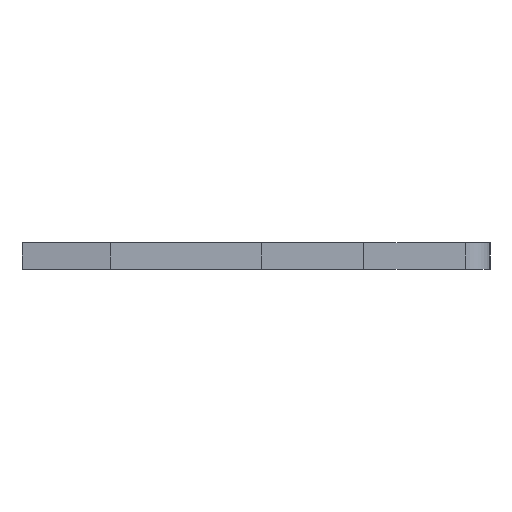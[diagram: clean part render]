
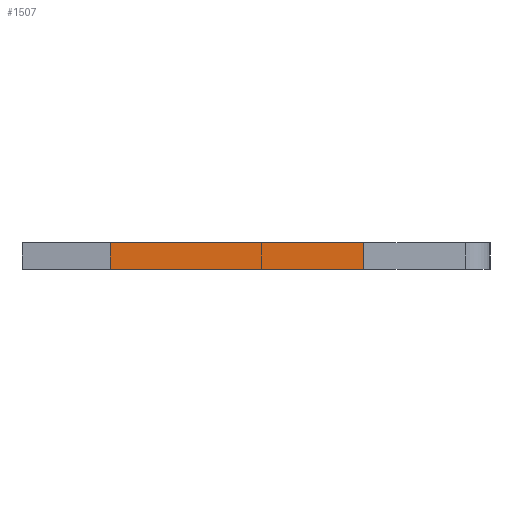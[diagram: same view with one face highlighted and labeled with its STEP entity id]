
A CAD part, left-side view. The second image highlights one B-rep face of the part: STEP entity #1507.
In plain terms, the highlighted face is planar.
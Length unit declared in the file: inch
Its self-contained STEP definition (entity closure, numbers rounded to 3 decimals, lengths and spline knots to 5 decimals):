
#182 = ORIENTED_EDGE ( 'NONE', *, *, #1383, .F. ) ;
#221 = CARTESIAN_POINT ( 'NONE',  ( 0.013, -0.099, -0.0575 ) ) ;
#313 = EDGE_LOOP ( 'NONE', ( #1690, #182, #1790, #849 ) ) ;
#319 = DIRECTION ( 'NONE',  ( 0., 1., 0. ) ) ;
#337 = CARTESIAN_POINT ( 'NONE',  ( -0.013, 0.146, -0.0575 ) ) ;
#366 = CARTESIAN_POINT ( 'NONE',  ( 0.013, 0.146, -0.0575 ) ) ;
#397 = DIRECTION ( 'NONE',  ( -1., 0., 0. ) ) ;
#422 = FACE_OUTER_BOUND ( 'NONE', #313, .T. ) ;
#446 = VECTOR ( 'NONE', #1350, 39.37008 ) ;
#530 = VERTEX_POINT ( 'NONE', #821 ) ;
#560 = DIRECTION ( 'NONE',  ( 1., 0., 0. ) ) ;
#689 = CARTESIAN_POINT ( 'NONE',  ( 0.013, -0.099, -0.0575 ) ) ;
#758 = VERTEX_POINT ( 'NONE', #1055 ) ;
#782 = VECTOR ( 'NONE', #1108, 39.37008 ) ;
#784 = EDGE_CURVE ( 'NONE', #2197, #758, #1020, .T. ) ;
#821 = CARTESIAN_POINT ( 'NONE',  ( 0.013, 0.146, -0.0575 ) ) ;
#849 = ORIENTED_EDGE ( 'NONE', *, *, #1523, .T. ) ;
#853 = VERTEX_POINT ( 'NONE', #689 ) ;
#1020 = LINE ( 'NONE', #337, #1537 ) ;
#1055 = CARTESIAN_POINT ( 'NONE',  ( -0.013, 0.146, -0.0575 ) ) ;
#1108 = DIRECTION ( 'NONE',  ( 0., 1., 0. ) ) ;
#1113 = LINE ( 'NONE', #366, #782 ) ;
#1190 = LINE ( 'NONE', #1676, #1817 ) ;
#1204 = AXIS2_PLACEMENT_3D ( 'NONE', #1330, #2236, #560 ) ;
#1261 = EDGE_CURVE ( 'NONE', #853, #530, #1113, .T. ) ;
#1330 = CARTESIAN_POINT ( 'NONE',  ( 0.013, 0.146, -0.0575 ) ) ;
#1350 = DIRECTION ( 'NONE',  ( -1., 0., 0. ) ) ;
#1383 = EDGE_CURVE ( 'NONE', #530, #758, #1190, .T. ) ;
#1507 = ADVANCED_FACE ( 'NONE', ( #422 ), #1522, .F. ) ;
#1522 = PLANE ( 'NONE',  #1204 ) ;
#1523 = EDGE_CURVE ( 'NONE', #853, #2197, #2138, .T. ) ;
#1537 = VECTOR ( 'NONE', #319, 39.37008 ) ;
#1676 = CARTESIAN_POINT ( 'NONE',  ( 0.013, 0.146, -0.0575 ) ) ;
#1690 = ORIENTED_EDGE ( 'NONE', *, *, #784, .T. ) ;
#1766 = CARTESIAN_POINT ( 'NONE',  ( -0.013, -0.099, -0.0575 ) ) ;
#1790 = ORIENTED_EDGE ( 'NONE', *, *, #1261, .F. ) ;
#1817 = VECTOR ( 'NONE', #397, 39.37008 ) ;
#2138 = LINE ( 'NONE', #221, #446 ) ;
#2197 = VERTEX_POINT ( 'NONE', #1766 ) ;
#2236 = DIRECTION ( 'NONE',  ( 0., 0., 1. ) ) ;
